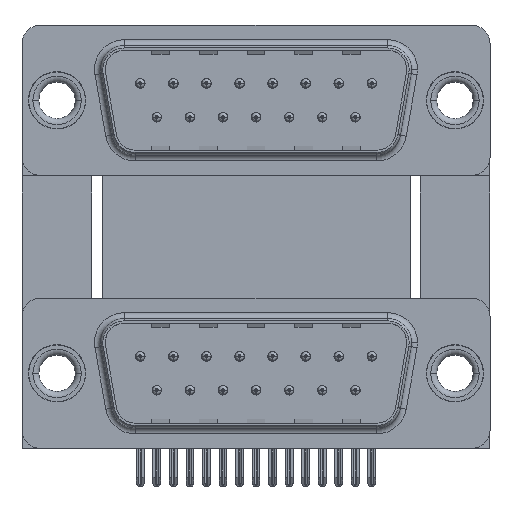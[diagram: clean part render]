
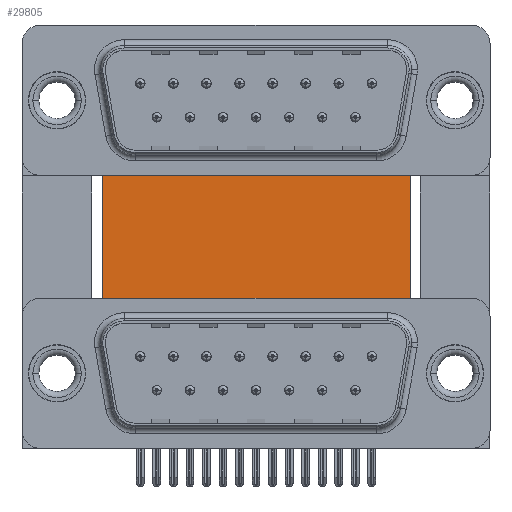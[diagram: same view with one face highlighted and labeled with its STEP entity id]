
A CAD part, top view. The second image highlights one B-rep face of the part: STEP entity #29805.
In plain terms, the highlighted planar face has unit normal (0, 0, 1).
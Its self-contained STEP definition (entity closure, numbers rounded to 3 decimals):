
#482 = CARTESIAN_POINT ( 'NONE',  ( 3.79, 16.585, -12. ) ) ;
#1216 = PLANE ( 'NONE',  #14523 ) ;
#4525 = DIRECTION ( 'NONE',  ( 1., 0., 0. ) ) ;
#5110 = ORIENTED_EDGE ( 'NONE', *, *, #16890, .T. ) ;
#6295 = CARTESIAN_POINT ( 'NONE',  ( 29.58, 16.585, -12. ) ) ;
#7421 = VECTOR ( 'NONE', #4525, 1000. ) ;
#7562 = LINE ( 'NONE', #20063, #16552 ) ;
#7949 = DIRECTION ( 'NONE',  ( -1., 0., 0. ) ) ;
#8609 = CARTESIAN_POINT ( 'NONE',  ( 3.79, -3.735, -12. ) ) ;
#8702 = VECTOR ( 'NONE', #11591, 1000. ) ;
#9062 = LINE ( 'NONE', #13970, #8702 ) ;
#10199 = VERTEX_POINT ( 'NONE', #482 ) ;
#11109 = VERTEX_POINT ( 'NONE', #17351 ) ;
#11591 = DIRECTION ( 'NONE',  ( 0., -1., 0. ) ) ;
#12236 = EDGE_CURVE ( 'NONE', #10199, #16673, #14357, .T. ) ;
#13807 = ORIENTED_EDGE ( 'NONE', *, *, #22752, .T. ) ;
#13970 = CARTESIAN_POINT ( 'NONE',  ( 3.79, 16.585, -12. ) ) ;
#14357 = LINE ( 'NONE', #31331, #22477 ) ;
#14523 = AXIS2_PLACEMENT_3D ( 'NONE', #27756, #30138, #7949 ) ;
#16552 = VECTOR ( 'NONE', #17231, 1000. ) ;
#16673 = VERTEX_POINT ( 'NONE', #6295 ) ;
#16890 = EDGE_CURVE ( 'NONE', #30667, #11109, #24070, .T. ) ;
#17231 = DIRECTION ( 'NONE',  ( 0., -1., 0. ) ) ;
#17351 = CARTESIAN_POINT ( 'NONE',  ( 29.58, -3.735, -12. ) ) ;
#19113 = ORIENTED_EDGE ( 'NONE', *, *, #12236, .F. ) ;
#20063 = CARTESIAN_POINT ( 'NONE',  ( 29.58, 16.585, -12. ) ) ;
#22477 = VECTOR ( 'NONE', #24041, 1000. ) ;
#22752 = EDGE_CURVE ( 'NONE', #10199, #30667, #9062, .T. ) ;
#23590 = CARTESIAN_POINT ( 'NONE',  ( 3.79, -3.735, -12. ) ) ;
#24041 = DIRECTION ( 'NONE',  ( 1., 0., 0. ) ) ;
#24070 = LINE ( 'NONE', #23590, #7421 ) ;
#27158 = ORIENTED_EDGE ( 'NONE', *, *, #30062, .F. ) ;
#27756 = CARTESIAN_POINT ( 'NONE',  ( 3.79, 16.585, -12. ) ) ;
#28317 = EDGE_LOOP ( 'NONE', ( #5110, #27158, #19113, #13807 ) ) ;
#29675 = FACE_OUTER_BOUND ( 'NONE', #28317, .T. ) ;
#29805 = ADVANCED_FACE ( 'NONE', ( #29675 ), #1216, .F. ) ;
#30062 = EDGE_CURVE ( 'NONE', #16673, #11109, #7562, .T. ) ;
#30138 = DIRECTION ( 'NONE',  ( 0., 0., -1. ) ) ;
#30667 = VERTEX_POINT ( 'NONE', #8609 ) ;
#31331 = CARTESIAN_POINT ( 'NONE',  ( 3.79, 16.585, -12. ) ) ;
